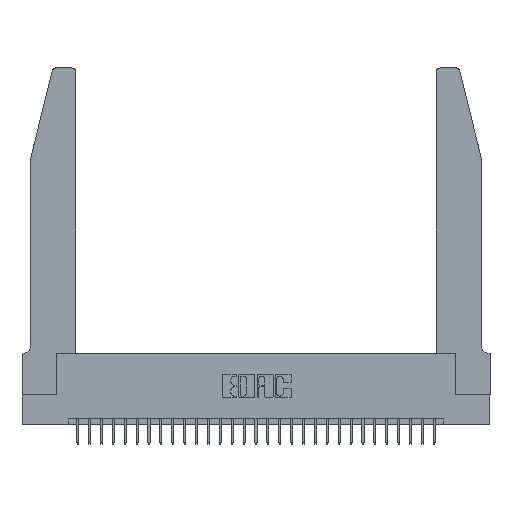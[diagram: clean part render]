
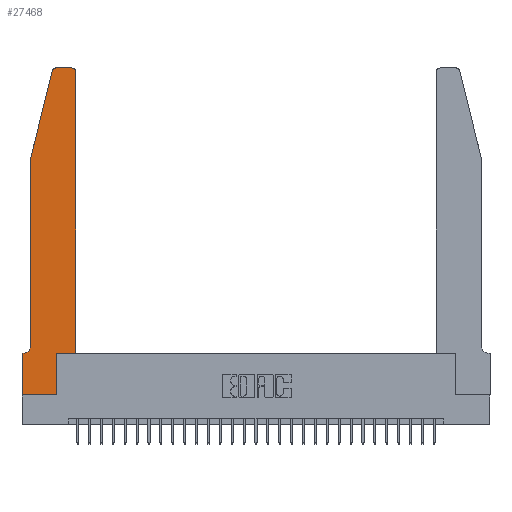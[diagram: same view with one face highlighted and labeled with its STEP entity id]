
A CAD part, top view. The second image highlights one B-rep face of the part: STEP entity #27468.
In plain terms, the highlighted planar face has unit normal (0, 0, 1).
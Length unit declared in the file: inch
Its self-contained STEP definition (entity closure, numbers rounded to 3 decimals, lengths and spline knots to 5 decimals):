
#935 = EDGE_CURVE ( 'NONE', #5781, #21440, #28708, .T. ) ;
#1074 = EDGE_CURVE ( 'NONE', #3432, #28123, #2446, .T. ) ;
#1365 = VERTEX_POINT ( 'NONE', #7106 ) ;
#1604 = EDGE_CURVE ( 'NONE', #16280, #5999, #22790, .T. ) ;
#2446 = LINE ( 'NONE', #14988, #20270 ) ;
#2571 = EDGE_CURVE ( 'NONE', #19680, #3432, #5717, .T. ) ;
#2612 = CARTESIAN_POINT ( 'NONE',  ( 0.2865, 0., 0.37 ) ) ;
#2789 = VECTOR ( 'NONE', #21354, 39.37008 ) ;
#3432 = VERTEX_POINT ( 'NONE', #27696 ) ;
#3649 = ORIENTED_EDGE ( 'NONE', *, *, #2571, .T. ) ;
#3850 = DIRECTION ( 'NONE',  ( 0., 1., 0. ) ) ;
#3873 = ORIENTED_EDGE ( 'NONE', *, *, #25155, .T. ) ;
#3879 = VECTOR ( 'NONE', #18388, 39.37008 ) ;
#3937 = DIRECTION ( 'NONE',  ( -1., 0., 0. ) ) ;
#3943 = CARTESIAN_POINT ( 'NONE',  ( 0.0755, 0.42, 0.37 ) ) ;
#5047 = VECTOR ( 'NONE', #22461, 39.37008 ) ;
#5304 = ORIENTED_EDGE ( 'NONE', *, *, #18686, .T. ) ;
#5717 = LINE ( 'NONE', #11156, #3879 ) ;
#5781 = VERTEX_POINT ( 'NONE', #17151 ) ;
#5999 = VERTEX_POINT ( 'NONE', #3943 ) ;
#6396 = DIRECTION ( 'NONE',  ( 0., 0., 1. ) ) ;
#6785 = LINE ( 'NONE', #17309, #29730 ) ;
#6864 = ORIENTED_EDGE ( 'NONE', *, *, #935, .T. ) ;
#7017 = CARTESIAN_POINT ( 'NONE',  ( 0.0755, 0.35, 0.37 ) ) ;
#7106 = CARTESIAN_POINT ( 'NONE',  ( 0.4205, 2.75, 0.37 ) ) ;
#7272 = FACE_OUTER_BOUND ( 'NONE', #15626, .T. ) ;
#7487 = ORIENTED_EDGE ( 'NONE', *, *, #1074, .T. ) ;
#7722 = DIRECTION ( 'NONE',  ( -1., 0., 0. ) ) ;
#8266 = LINE ( 'NONE', #30093, #24917 ) ;
#8398 = CARTESIAN_POINT ( 'NONE',  ( 0.4505, 0.35, 0.37 ) ) ;
#8702 = CARTESIAN_POINT ( 'NONE',  ( 0.0055, 0.42, 0.37 ) ) ;
#8886 = ORIENTED_EDGE ( 'NONE', *, *, #18858, .T. ) ;
#9387 = EDGE_CURVE ( 'NONE', #11070, #19680, #19640, .T. ) ;
#9480 = ORIENTED_EDGE ( 'NONE', *, *, #24089, .T. ) ;
#10124 = DIRECTION ( 'NONE',  ( 0., 0., 1. ) ) ;
#10805 = CIRCLE ( 'NONE', #23556, 0.03 ) ;
#10902 = CARTESIAN_POINT ( 'NONE',  ( 0.0755, 2., 0.37 ) ) ;
#11070 = VERTEX_POINT ( 'NONE', #19899 ) ;
#11156 = CARTESIAN_POINT ( 'NONE',  ( 0.2865, 0.35, 0.37 ) ) ;
#11376 = CIRCLE ( 'NONE', #15859, 0.03 ) ;
#11676 = ORIENTED_EDGE ( 'NONE', *, *, #25534, .T. ) ;
#11916 = DIRECTION ( 'NONE',  ( 1., 0., 0. ) ) ;
#12202 = CARTESIAN_POINT ( 'NONE',  ( 0., 0.35, 0.37 ) ) ;
#12218 = CARTESIAN_POINT ( 'NONE',  ( 0.0755, 2., 0.37 ) ) ;
#12618 = CARTESIAN_POINT ( 'NONE',  ( 0.2605, 2.75, 0.37 ) ) ;
#13359 = CARTESIAN_POINT ( 'NONE',  ( 0.4205, 2.72, 0.37 ) ) ;
#13599 = ORIENTED_EDGE ( 'NONE', *, *, #27987, .T. ) ;
#13760 = DIRECTION ( 'NONE',  ( 0., 0., -1. ) ) ;
#14904 = CARTESIAN_POINT ( 'NONE',  ( 0.4505, 0.35, 0.37 ) ) ;
#14988 = CARTESIAN_POINT ( 'NONE',  ( 0.4505, 0.35, 0.37 ) ) ;
#15060 = CARTESIAN_POINT ( 'NONE',  ( 0.284, 2.75, 0.37 ) ) ;
#15626 = EDGE_LOOP ( 'NONE', ( #11676, #13599, #9480, #18802, #8886, #6864, #5304, #28866, #3649, #7487, #28580, #3873 ) ) ;
#15859 = AXIS2_PLACEMENT_3D ( 'NONE', #21927, #26248, #28848 ) ;
#16146 = DIRECTION ( 'NONE',  ( -0.239, -0.971, 0. ) ) ;
#16280 = VERTEX_POINT ( 'NONE', #12218 ) ;
#16346 = CARTESIAN_POINT ( 'NONE',  ( 0., 0., 0.37 ) ) ;
#17105 = VERTEX_POINT ( 'NONE', #22900 ) ;
#17151 = CARTESIAN_POINT ( 'NONE',  ( 0.0055, 0.35, 0.37 ) ) ;
#17309 = CARTESIAN_POINT ( 'NONE',  ( 0., 0., 0.37 ) ) ;
#18133 = DIRECTION ( 'NONE',  ( 1., 0., 0. ) ) ;
#18388 = DIRECTION ( 'NONE',  ( 0., 1., 0. ) ) ;
#18502 = CARTESIAN_POINT ( 'NONE',  ( 0., 0.35, 0.37 ) ) ;
#18665 = CIRCLE ( 'NONE', #23218, 0.07 ) ;
#18686 = EDGE_CURVE ( 'NONE', #21440, #11070, #6785, .T. ) ;
#18802 = ORIENTED_EDGE ( 'NONE', *, *, #1604, .T. ) ;
#18858 = EDGE_CURVE ( 'NONE', #5999, #5781, #18665, .T. ) ;
#19248 = VECTOR ( 'NONE', #11916, 39.37008 ) ;
#19420 = PLANE ( 'NONE',  #22786 ) ;
#19640 = LINE ( 'NONE', #16346, #19248 ) ;
#19680 = VERTEX_POINT ( 'NONE', #2612 ) ;
#19899 = CARTESIAN_POINT ( 'NONE',  ( 0., 0., 0.37 ) ) ;
#20270 = VECTOR ( 'NONE', #27057, 39.37008 ) ;
#21120 = LINE ( 'NONE', #12618, #28852 ) ;
#21354 = DIRECTION ( 'NONE',  ( -1., 0., 0. ) ) ;
#21440 = VERTEX_POINT ( 'NONE', #18502 ) ;
#21927 = CARTESIAN_POINT ( 'NONE',  ( 0.284, 2.72, 0.37 ) ) ;
#22461 = DIRECTION ( 'NONE',  ( 0., -1., 0. ) ) ;
#22786 = AXIS2_PLACEMENT_3D ( 'NONE', #12202, #10124, #24289 ) ;
#22790 = LINE ( 'NONE', #10902, #5047 ) ;
#22900 = CARTESIAN_POINT ( 'NONE',  ( 0.4505, 2.72, 0.37 ) ) ;
#22999 = VERTEX_POINT ( 'NONE', #15060 ) ;
#23218 = AXIS2_PLACEMENT_3D ( 'NONE', #8702, #13760, #3937 ) ;
#23556 = AXIS2_PLACEMENT_3D ( 'NONE', #13359, #6396, #18133 ) ;
#23996 = EDGE_CURVE ( 'NONE', #28123, #17105, #30443, .T. ) ;
#24089 = EDGE_CURVE ( 'NONE', #24980, #16280, #8266, .T. ) ;
#24289 = DIRECTION ( 'NONE',  ( 1., 0., 0. ) ) ;
#24917 = VECTOR ( 'NONE', #16146, 39.37008 ) ;
#24980 = VERTEX_POINT ( 'NONE', #27084 ) ;
#25155 = EDGE_CURVE ( 'NONE', #17105, #1365, #10805, .T. ) ;
#25534 = EDGE_CURVE ( 'NONE', #1365, #22999, #21120, .T. ) ;
#26248 = DIRECTION ( 'NONE',  ( 0., 0., 1. ) ) ;
#27057 = DIRECTION ( 'NONE',  ( 1., 0., 0. ) ) ;
#27084 = CARTESIAN_POINT ( 'NONE',  ( 0.25487, 2.72718, 0.37 ) ) ;
#27468 = ADVANCED_FACE ( 'NONE', ( #7272 ), #19420, .T. ) ;
#27696 = CARTESIAN_POINT ( 'NONE',  ( 0.2865, 0.35, 0.37 ) ) ;
#27987 = EDGE_CURVE ( 'NONE', #22999, #24980, #11376, .T. ) ;
#28123 = VERTEX_POINT ( 'NONE', #14904 ) ;
#28580 = ORIENTED_EDGE ( 'NONE', *, *, #23996, .T. ) ;
#28586 = VECTOR ( 'NONE', #3850, 39.37008 ) ;
#28708 = LINE ( 'NONE', #7017, #2789 ) ;
#28848 = DIRECTION ( 'NONE',  ( 1., 0., 0. ) ) ;
#28852 = VECTOR ( 'NONE', #7722, 39.37008 ) ;
#28866 = ORIENTED_EDGE ( 'NONE', *, *, #9387, .T. ) ;
#28871 = DIRECTION ( 'NONE',  ( 0., -1., 0. ) ) ;
#29730 = VECTOR ( 'NONE', #28871, 39.37008 ) ;
#30093 = CARTESIAN_POINT ( 'NONE',  ( 0.0755, 2., 0.37 ) ) ;
#30443 = LINE ( 'NONE', #8398, #28586 ) ;
